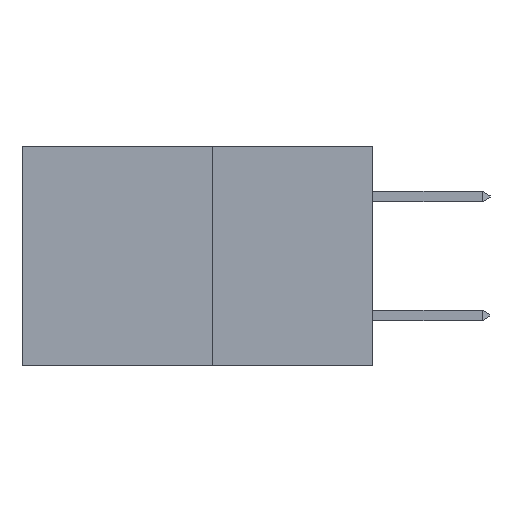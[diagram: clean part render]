
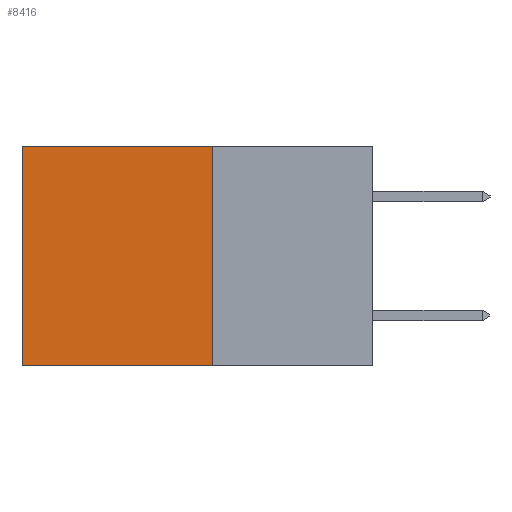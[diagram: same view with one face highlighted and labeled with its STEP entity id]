
A CAD part, left-side view. The second image highlights one B-rep face of the part: STEP entity #8416.
In plain terms, the highlighted planar face has unit normal (-1, 0, 0).
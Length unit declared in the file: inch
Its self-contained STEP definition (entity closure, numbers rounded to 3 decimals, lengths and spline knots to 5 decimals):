
#179 = CARTESIAN_POINT ( 'NONE',  ( 0.277, 0.59, 0. ) ) ;
#286 = CARTESIAN_POINT ( 'NONE',  ( 0.277, 0.27, 0. ) ) ;
#604 = EDGE_CURVE ( 'NONE', #6485, #4451, #6879, .T. ) ;
#2324 = FACE_OUTER_BOUND ( 'NONE', #6302, .T. ) ;
#2849 = DIRECTION ( 'NONE',  ( 0., 1., 0. ) ) ;
#2873 = CARTESIAN_POINT ( 'NONE',  ( 0.277, 0.59, -0.37 ) ) ;
#3803 = DIRECTION ( 'NONE',  ( 0., 0., -1. ) ) ;
#3847 = VECTOR ( 'NONE', #2849, 39.37008 ) ;
#3865 = ORIENTED_EDGE ( 'NONE', *, *, #12395, .T. ) ;
#3873 = CARTESIAN_POINT ( 'NONE',  ( 0.277, 0.27, -0.37 ) ) ;
#3940 = DIRECTION ( 'NONE',  ( 0., 0., -1. ) ) ;
#4333 = VECTOR ( 'NONE', #3940, 39.37008 ) ;
#4451 = VERTEX_POINT ( 'NONE', #179 ) ;
#4516 = VERTEX_POINT ( 'NONE', #12212 ) ;
#5530 = EDGE_CURVE ( 'NONE', #4516, #6707, #8719, .T. ) ;
#5860 = VECTOR ( 'NONE', #10016, 39.37008 ) ;
#6302 = EDGE_LOOP ( 'NONE', ( #3865, #9079, #11430, #11443 ) ) ;
#6485 = VERTEX_POINT ( 'NONE', #9824 ) ;
#6707 = VERTEX_POINT ( 'NONE', #8250 ) ;
#6879 = LINE ( 'NONE', #286, #3847 ) ;
#7055 = LINE ( 'NONE', #2873, #4333 ) ;
#7405 = EDGE_CURVE ( 'NONE', #6485, #4516, #12205, .T. ) ;
#8250 = CARTESIAN_POINT ( 'NONE',  ( 0.277, 0.59, -0.37 ) ) ;
#8416 = ADVANCED_FACE ( 'NONE', ( #2324 ), #10938, .F. ) ;
#8719 = LINE ( 'NONE', #9963, #5860 ) ;
#9079 = ORIENTED_EDGE ( 'NONE', *, *, #5530, .F. ) ;
#9729 = VECTOR ( 'NONE', #3803, 39.37008 ) ;
#9824 = CARTESIAN_POINT ( 'NONE',  ( 0.277, 0.27, 0. ) ) ;
#9963 = CARTESIAN_POINT ( 'NONE',  ( 0.277, 0.27, -0.37 ) ) ;
#10016 = DIRECTION ( 'NONE',  ( 0., 1., 0. ) ) ;
#10134 = DIRECTION ( 'NONE',  ( 0., 0., -1. ) ) ;
#10227 = DIRECTION ( 'NONE',  ( 1., 0., 0. ) ) ;
#10938 = PLANE ( 'NONE',  #12667 ) ;
#11430 = ORIENTED_EDGE ( 'NONE', *, *, #7405, .F. ) ;
#11443 = ORIENTED_EDGE ( 'NONE', *, *, #604, .T. ) ;
#12205 = LINE ( 'NONE', #3873, #9729 ) ;
#12212 = CARTESIAN_POINT ( 'NONE',  ( 0.277, 0.27, -0.37 ) ) ;
#12395 = EDGE_CURVE ( 'NONE', #4451, #6707, #7055, .T. ) ;
#12667 = AXIS2_PLACEMENT_3D ( 'NONE', #12674, #10227, #10134 ) ;
#12674 = CARTESIAN_POINT ( 'NONE',  ( 0.277, 0.27, -0.37 ) ) ;
